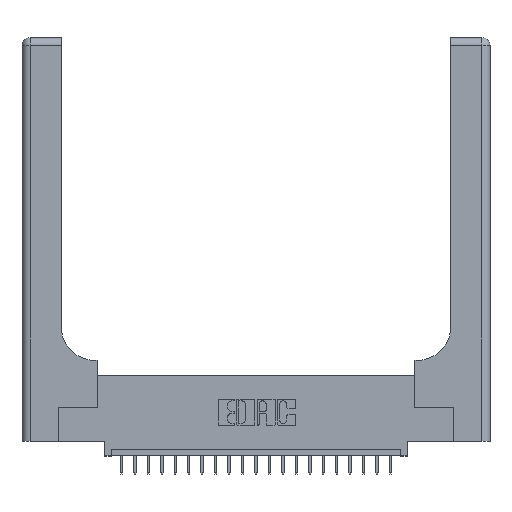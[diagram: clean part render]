
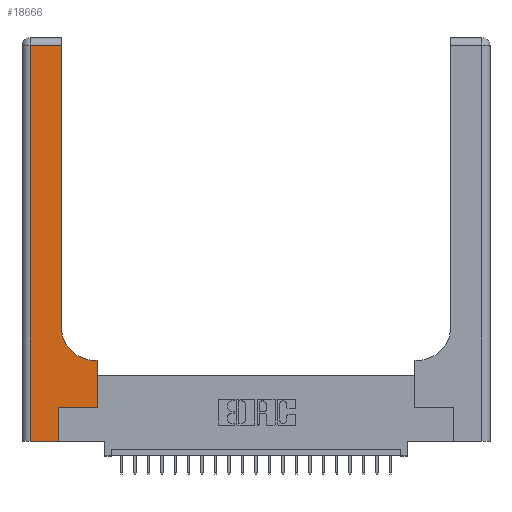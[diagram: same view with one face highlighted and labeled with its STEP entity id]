
A CAD part, top view. The second image highlights one B-rep face of the part: STEP entity #18666.
In plain terms, the highlighted planar face has unit normal (0, 0, 1).
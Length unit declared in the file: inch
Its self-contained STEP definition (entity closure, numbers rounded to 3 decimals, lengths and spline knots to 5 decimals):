
#67 = EDGE_LOOP ( 'NONE', ( #18831, #19347, #10952, #12634, #3113, #20664, #20641, #16754, #8158 ) ) ;
#76 = PLANE ( 'NONE',  #5219 ) ;
#808 = LINE ( 'NONE', #8124, #23596 ) ;
#892 = VECTOR ( 'NONE', #3632, 39.37008 ) ;
#1192 = LINE ( 'NONE', #12709, #14629 ) ;
#1402 = LINE ( 'NONE', #17871, #12224 ) ;
#1519 = EDGE_CURVE ( 'NONE', #10211, #19162, #14832, .T. ) ;
#1561 = EDGE_CURVE ( 'NONE', #9030, #10260, #20665, .T. ) ;
#1669 = CARTESIAN_POINT ( 'NONE',  ( 0., 2.94, 0.37 ) ) ;
#3113 = ORIENTED_EDGE ( 'NONE', *, *, #7033, .T. ) ;
#3632 = DIRECTION ( 'NONE',  ( 1., 0., 0. ) ) ;
#3989 = VERTEX_POINT ( 'NONE', #21944 ) ;
#4088 = VERTEX_POINT ( 'NONE', #22894 ) ;
#4986 = DIRECTION ( 'NONE',  ( 0., -1., 0. ) ) ;
#5219 = AXIS2_PLACEMENT_3D ( 'NONE', #14941, #22365, #18376 ) ;
#6077 = CIRCLE ( 'NONE', #9587, 0.25 ) ;
#7033 = EDGE_CURVE ( 'NONE', #10260, #3989, #1402, .T. ) ;
#8006 = VECTOR ( 'NONE', #22797, 39.37008 ) ;
#8124 = CARTESIAN_POINT ( 'NONE',  ( 0.2915, 3., 0.37 ) ) ;
#8145 = CARTESIAN_POINT ( 'NONE',  ( 0.5585, 0.6, 0.37 ) ) ;
#8158 = ORIENTED_EDGE ( 'NONE', *, *, #11071, .T. ) ;
#8204 = CARTESIAN_POINT ( 'NONE',  ( 0.06, 2.94, 0.37 ) ) ;
#8434 = VERTEX_POINT ( 'NONE', #20507 ) ;
#8987 = DIRECTION ( 'NONE',  ( -1., 0., 0. ) ) ;
#9030 = VERTEX_POINT ( 'NONE', #17982 ) ;
#9479 = CARTESIAN_POINT ( 'NONE',  ( 0., 0., 0.37 ) ) ;
#9510 = VECTOR ( 'NONE', #4986, 39.37008 ) ;
#9587 = AXIS2_PLACEMENT_3D ( 'NONE', #16783, #11304, #22369 ) ;
#10135 = LINE ( 'NONE', #14126, #9510 ) ;
#10136 = CARTESIAN_POINT ( 'NONE',  ( 0.2915, 2.94, 0.37 ) ) ;
#10211 = VERTEX_POINT ( 'NONE', #10136 ) ;
#10260 = VERTEX_POINT ( 'NONE', #12572 ) ;
#10710 = EDGE_CURVE ( 'NONE', #16795, #8434, #15398, .T. ) ;
#10952 = ORIENTED_EDGE ( 'NONE', *, *, #16518, .T. ) ;
#10972 = LINE ( 'NONE', #14849, #892 ) ;
#11071 = EDGE_CURVE ( 'NONE', #8434, #14648, #6077, .T. ) ;
#11304 = DIRECTION ( 'NONE',  ( 0., 0., -1. ) ) ;
#12224 = VECTOR ( 'NONE', #18117, 39.37008 ) ;
#12572 = CARTESIAN_POINT ( 'NONE',  ( 0.269, 0., 0.37 ) ) ;
#12634 = ORIENTED_EDGE ( 'NONE', *, *, #1561, .T. ) ;
#12709 = CARTESIAN_POINT ( 'NONE',  ( 0.5585, 0.25, 0.37 ) ) ;
#13583 = CARTESIAN_POINT ( 'NONE',  ( 0.2915, 0.6, 0.37 ) ) ;
#14126 = CARTESIAN_POINT ( 'NONE',  ( 0.06, 3., 0.37 ) ) ;
#14629 = VECTOR ( 'NONE', #20094, 39.37008 ) ;
#14648 = VERTEX_POINT ( 'NONE', #18260 ) ;
#14832 = LINE ( 'NONE', #1669, #19862 ) ;
#14849 = CARTESIAN_POINT ( 'NONE',  ( 0.269, 0.25, 0.37 ) ) ;
#14941 = CARTESIAN_POINT ( 'NONE',  ( 0., 3., 0.37 ) ) ;
#15398 = LINE ( 'NONE', #13583, #8006 ) ;
#15561 = EDGE_CURVE ( 'NONE', #3989, #4088, #10972, .T. ) ;
#16518 = EDGE_CURVE ( 'NONE', #19162, #9030, #10135, .T. ) ;
#16754 = ORIENTED_EDGE ( 'NONE', *, *, #10710, .T. ) ;
#16777 = FACE_OUTER_BOUND ( 'NONE', #67, .T. ) ;
#16783 = CARTESIAN_POINT ( 'NONE',  ( 0.5415, 0.85, 0.37 ) ) ;
#16795 = VERTEX_POINT ( 'NONE', #8145 ) ;
#17871 = CARTESIAN_POINT ( 'NONE',  ( 0.269, 0., 0.37 ) ) ;
#17982 = CARTESIAN_POINT ( 'NONE',  ( 0.06, 0., 0.37 ) ) ;
#18117 = DIRECTION ( 'NONE',  ( 0., 1., 0. ) ) ;
#18260 = CARTESIAN_POINT ( 'NONE',  ( 0.2915, 0.85, 0.37 ) ) ;
#18376 = DIRECTION ( 'NONE',  ( -1., 0., 0. ) ) ;
#18666 = ADVANCED_FACE ( 'NONE', ( #16777 ), #76, .F. ) ;
#18831 = ORIENTED_EDGE ( 'NONE', *, *, #22367, .T. ) ;
#19162 = VERTEX_POINT ( 'NONE', #8204 ) ;
#19347 = ORIENTED_EDGE ( 'NONE', *, *, #1519, .T. ) ;
#19862 = VECTOR ( 'NONE', #8987, 39.37008 ) ;
#20094 = DIRECTION ( 'NONE',  ( 0., 1., 0. ) ) ;
#20507 = CARTESIAN_POINT ( 'NONE',  ( 0.5415, 0.6, 0.37 ) ) ;
#20641 = ORIENTED_EDGE ( 'NONE', *, *, #20761, .T. ) ;
#20643 = VECTOR ( 'NONE', #23800, 39.37008 ) ;
#20664 = ORIENTED_EDGE ( 'NONE', *, *, #15561, .T. ) ;
#20665 = LINE ( 'NONE', #9479, #20643 ) ;
#20761 = EDGE_CURVE ( 'NONE', #4088, #16795, #1192, .T. ) ;
#21493 = DIRECTION ( 'NONE',  ( 0., 1., 0. ) ) ;
#21944 = CARTESIAN_POINT ( 'NONE',  ( 0.269, 0.25, 0.37 ) ) ;
#22365 = DIRECTION ( 'NONE',  ( 0., 0., -1. ) ) ;
#22367 = EDGE_CURVE ( 'NONE', #14648, #10211, #808, .T. ) ;
#22369 = DIRECTION ( 'NONE',  ( 1., 0., 0. ) ) ;
#22797 = DIRECTION ( 'NONE',  ( -1., 0., 0. ) ) ;
#22894 = CARTESIAN_POINT ( 'NONE',  ( 0.5585, 0.25, 0.37 ) ) ;
#23596 = VECTOR ( 'NONE', #21493, 39.37008 ) ;
#23800 = DIRECTION ( 'NONE',  ( 1., 0., 0. ) ) ;
